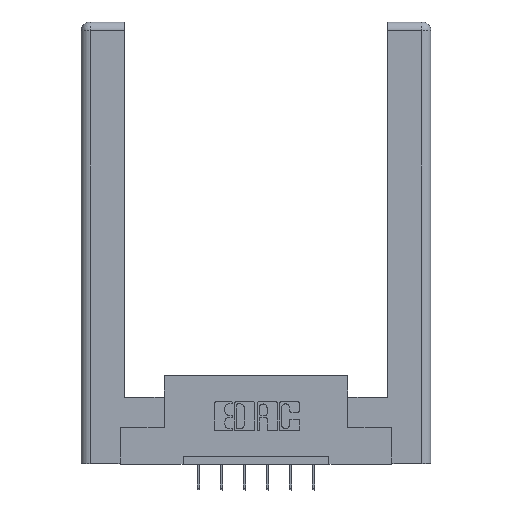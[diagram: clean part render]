
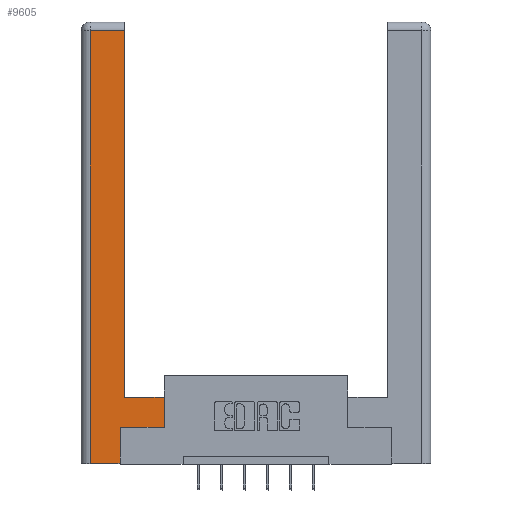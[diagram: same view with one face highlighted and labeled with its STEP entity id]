
A CAD part, top view. The second image highlights one B-rep face of the part: STEP entity #9605.
In plain terms, the highlighted planar face has unit normal (0, 0, 1).
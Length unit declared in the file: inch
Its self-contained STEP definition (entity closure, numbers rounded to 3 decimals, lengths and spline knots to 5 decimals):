
#105 = CARTESIAN_POINT ( 'NONE',  ( 0.265, 0.245, 0. ) ) ;
#281 = VECTOR ( 'NONE', #6806, 39.37008 ) ;
#291 = VECTOR ( 'NONE', #6105, 39.37008 ) ;
#510 = CARTESIAN_POINT ( 'NONE',  ( 0.265, 0.245, 0. ) ) ;
#859 = VERTEX_POINT ( 'NONE', #6463 ) ;
#1205 = CARTESIAN_POINT ( 'NONE',  ( 0.0615, 0., 0. ) ) ;
#1673 = VERTEX_POINT ( 'NONE', #6888 ) ;
#1697 = LINE ( 'NONE', #11571, #10138 ) ;
#1732 = EDGE_CURVE ( 'NONE', #859, #6283, #1844, .T. ) ;
#1844 = LINE ( 'NONE', #510, #11582 ) ;
#1938 = DIRECTION ( 'NONE',  ( 0., 1., 0. ) ) ;
#2277 = ORIENTED_EDGE ( 'NONE', *, *, #1732, .T. ) ;
#2453 = DIRECTION ( 'NONE',  ( 0., 0., -1. ) ) ;
#2662 = CARTESIAN_POINT ( 'NONE',  ( 0.565, 0.45, 0. ) ) ;
#2836 = VECTOR ( 'NONE', #10357, 39.37008 ) ;
#3033 = CARTESIAN_POINT ( 'NONE',  ( 0.295, 0.45, 0. ) ) ;
#3294 = VECTOR ( 'NONE', #9997, 39.37008 ) ;
#3370 = ORIENTED_EDGE ( 'NONE', *, *, #8217, .T. ) ;
#3374 = DIRECTION ( 'NONE',  ( -1., 0., 0. ) ) ;
#3397 = EDGE_CURVE ( 'NONE', #5909, #1673, #9107, .T. ) ;
#3491 = VERTEX_POINT ( 'NONE', #8979 ) ;
#3506 = ORIENTED_EDGE ( 'NONE', *, *, #8264, .T. ) ;
#4157 = VERTEX_POINT ( 'NONE', #3033 ) ;
#4234 = VECTOR ( 'NONE', #5286, 39.37008 ) ;
#4369 = CARTESIAN_POINT ( 'NONE',  ( 0., 0., 0. ) ) ;
#4801 = EDGE_CURVE ( 'NONE', #6683, #6730, #8793, .T. ) ;
#4994 = FACE_OUTER_BOUND ( 'NONE', #10630, .T. ) ;
#5203 = ORIENTED_EDGE ( 'NONE', *, *, #4801, .T. ) ;
#5260 = DIRECTION ( 'NONE',  ( 0., 1., 0. ) ) ;
#5286 = DIRECTION ( 'NONE',  ( 0., 1., 0. ) ) ;
#5909 = VERTEX_POINT ( 'NONE', #10973 ) ;
#6003 = CARTESIAN_POINT ( 'NONE',  ( 0.565, 0.245, 0. ) ) ;
#6006 = VECTOR ( 'NONE', #10389, 39.37008 ) ;
#6105 = DIRECTION ( 'NONE',  ( 1., 0., 0. ) ) ;
#6283 = VERTEX_POINT ( 'NONE', #105 ) ;
#6463 = CARTESIAN_POINT ( 'NONE',  ( 0.265, 0., 0. ) ) ;
#6683 = VERTEX_POINT ( 'NONE', #6003 ) ;
#6730 = VERTEX_POINT ( 'NONE', #9204 ) ;
#6806 = DIRECTION ( 'NONE',  ( -1., 0., 0. ) ) ;
#6888 = CARTESIAN_POINT ( 'NONE',  ( 0.0615, 0., 0. ) ) ;
#6926 = CARTESIAN_POINT ( 'NONE',  ( 0.0615, 2.94, 0. ) ) ;
#7223 = ORIENTED_EDGE ( 'NONE', *, *, #9011, .T. ) ;
#7363 = ORIENTED_EDGE ( 'NONE', *, *, #3397, .T. ) ;
#7711 = LINE ( 'NONE', #10953, #3294 ) ;
#8157 = LINE ( 'NONE', #6926, #281 ) ;
#8217 = EDGE_CURVE ( 'NONE', #6730, #4157, #9290, .T. ) ;
#8264 = EDGE_CURVE ( 'NONE', #6283, #6683, #10597, .T. ) ;
#8312 = ORIENTED_EDGE ( 'NONE', *, *, #8683, .T. ) ;
#8662 = CARTESIAN_POINT ( 'NONE',  ( 0.565, 0.245, 0. ) ) ;
#8683 = EDGE_CURVE ( 'NONE', #3491, #5909, #8157, .T. ) ;
#8725 = AXIS2_PLACEMENT_3D ( 'NONE', #4369, #2453, #3374 ) ;
#8793 = LINE ( 'NONE', #2662, #4234 ) ;
#8917 = EDGE_CURVE ( 'NONE', #4157, #3491, #1697, .T. ) ;
#8979 = CARTESIAN_POINT ( 'NONE',  ( 0.295, 2.94, 0. ) ) ;
#9011 = EDGE_CURVE ( 'NONE', #1673, #859, #7711, .T. ) ;
#9107 = LINE ( 'NONE', #1205, #2836 ) ;
#9204 = CARTESIAN_POINT ( 'NONE',  ( 0.565, 0.45, 0. ) ) ;
#9205 = ORIENTED_EDGE ( 'NONE', *, *, #8917, .T. ) ;
#9290 = LINE ( 'NONE', #10668, #6006 ) ;
#9605 = ADVANCED_FACE ( 'NONE', ( #4994 ), #11720, .F. ) ;
#9997 = DIRECTION ( 'NONE',  ( 1., 0., 0. ) ) ;
#10138 = VECTOR ( 'NONE', #5260, 39.37008 ) ;
#10357 = DIRECTION ( 'NONE',  ( 0., -1., 0. ) ) ;
#10389 = DIRECTION ( 'NONE',  ( -1., 0., 0. ) ) ;
#10597 = LINE ( 'NONE', #8662, #291 ) ;
#10630 = EDGE_LOOP ( 'NONE', ( #9205, #8312, #7363, #7223, #2277, #3506, #5203, #3370 ) ) ;
#10668 = CARTESIAN_POINT ( 'NONE',  ( 0.295, 0.45, 0. ) ) ;
#10953 = CARTESIAN_POINT ( 'NONE',  ( 0.265, 0., 0. ) ) ;
#10973 = CARTESIAN_POINT ( 'NONE',  ( 0.0615, 2.94, 0. ) ) ;
#11571 = CARTESIAN_POINT ( 'NONE',  ( 0.295, 3., 0. ) ) ;
#11582 = VECTOR ( 'NONE', #1938, 39.37008 ) ;
#11720 = PLANE ( 'NONE',  #8725 ) ;
